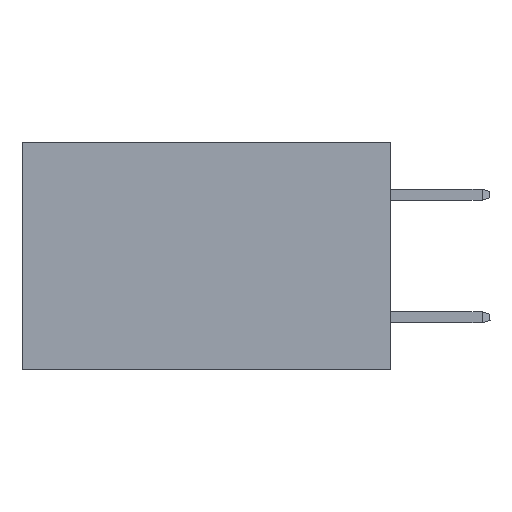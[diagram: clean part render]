
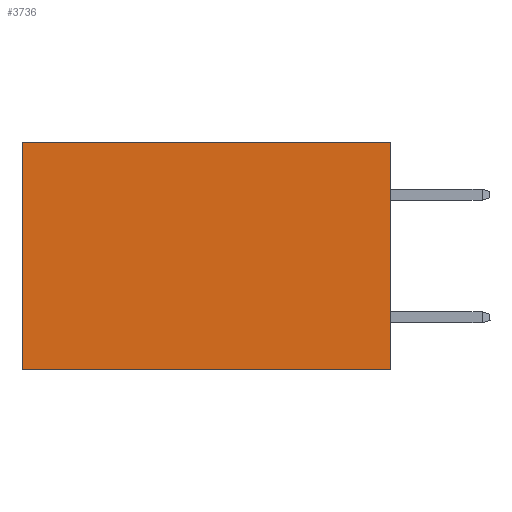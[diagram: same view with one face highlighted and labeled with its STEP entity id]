
A CAD part, left-side view. The second image highlights one B-rep face of the part: STEP entity #3736.
In plain terms, the highlighted planar face has unit normal (-1, 0, 0).
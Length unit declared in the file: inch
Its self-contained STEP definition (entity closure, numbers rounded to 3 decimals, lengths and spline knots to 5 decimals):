
#1606 = ORIENTED_EDGE ( 'NONE', *, *, #16791, .F. ) ;
#1943 = EDGE_CURVE ( 'NONE', #15106, #12204, #16857, .T. ) ;
#2524 = ORIENTED_EDGE ( 'NONE', *, *, #9430, .F. ) ;
#2599 = DIRECTION ( 'NONE',  ( 0., 0., -1. ) ) ;
#2858 = EDGE_LOOP ( 'NONE', ( #13224, #1606, #2524, #11033 ) ) ;
#3736 = ADVANCED_FACE ( 'NONE', ( #6759 ), #9290, .F. ) ;
#5315 = CARTESIAN_POINT ( 'NONE',  ( 0.2875, 0.6, 0. ) ) ;
#5897 = CARTESIAN_POINT ( 'NONE',  ( 0.2875, 0., 0. ) ) ;
#6490 = VECTOR ( 'NONE', #9851, 39.37008 ) ;
#6759 = FACE_OUTER_BOUND ( 'NONE', #2858, .T. ) ;
#8524 = LINE ( 'NONE', #11477, #6490 ) ;
#9290 = PLANE ( 'NONE',  #12730 ) ;
#9380 = DIRECTION ( 'NONE',  ( 0., 0., -1. ) ) ;
#9430 = EDGE_CURVE ( 'NONE', #15106, #19009, #15324, .T. ) ;
#9851 = DIRECTION ( 'NONE',  ( 0., 1., 0. ) ) ;
#11033 = ORIENTED_EDGE ( 'NONE', *, *, #1943, .T. ) ;
#11171 = CARTESIAN_POINT ( 'NONE',  ( 0.2875, 0., 0. ) ) ;
#11477 = CARTESIAN_POINT ( 'NONE',  ( 0.2875, 0., -0.37 ) ) ;
#11632 = DIRECTION ( 'NONE',  ( 0., 0., -1. ) ) ;
#11935 = CARTESIAN_POINT ( 'NONE',  ( 0.2875, 0., 0. ) ) ;
#12173 = DIRECTION ( 'NONE',  ( 0., 1., 0. ) ) ;
#12204 = VERTEX_POINT ( 'NONE', #5315 ) ;
#12321 = EDGE_CURVE ( 'NONE', #12204, #24071, #19972, .T. ) ;
#12730 = AXIS2_PLACEMENT_3D ( 'NONE', #11171, #18795, #11632 ) ;
#13224 = ORIENTED_EDGE ( 'NONE', *, *, #12321, .T. ) ;
#13538 = VECTOR ( 'NONE', #2599, 39.37008 ) ;
#14838 = CARTESIAN_POINT ( 'NONE',  ( 0.2875, 0.6, -0.37 ) ) ;
#15106 = VERTEX_POINT ( 'NONE', #11935 ) ;
#15324 = LINE ( 'NONE', #5897, #13538 ) ;
#16791 = EDGE_CURVE ( 'NONE', #19009, #24071, #8524, .T. ) ;
#16857 = LINE ( 'NONE', #23471, #20685 ) ;
#18795 = DIRECTION ( 'NONE',  ( 1., 0., 0. ) ) ;
#19009 = VERTEX_POINT ( 'NONE', #20916 ) ;
#19972 = LINE ( 'NONE', #24024, #22613 ) ;
#20685 = VECTOR ( 'NONE', #12173, 39.37008 ) ;
#20916 = CARTESIAN_POINT ( 'NONE',  ( 0.2875, 0., -0.37 ) ) ;
#22613 = VECTOR ( 'NONE', #9380, 39.37008 ) ;
#23471 = CARTESIAN_POINT ( 'NONE',  ( 0.2875, 0., 0. ) ) ;
#24024 = CARTESIAN_POINT ( 'NONE',  ( 0.2875, 0.6, 0. ) ) ;
#24071 = VERTEX_POINT ( 'NONE', #14838 ) ;
